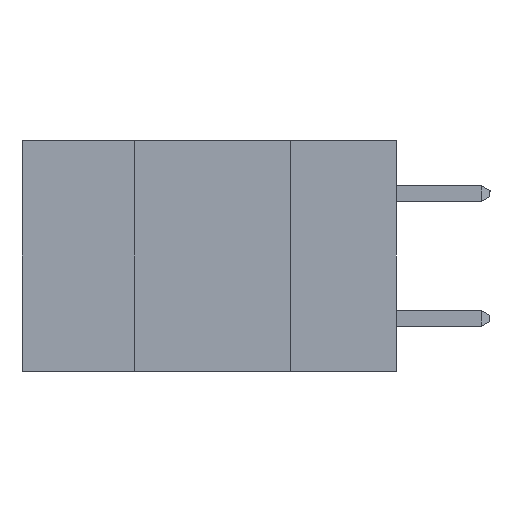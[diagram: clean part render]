
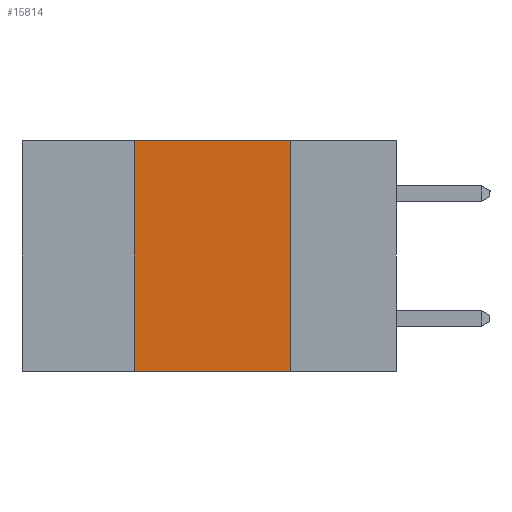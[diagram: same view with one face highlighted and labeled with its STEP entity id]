
A CAD part, left-side view. The second image highlights one B-rep face of the part: STEP entity #15814.
In plain terms, the highlighted planar face has unit normal (-1, 0, 0).
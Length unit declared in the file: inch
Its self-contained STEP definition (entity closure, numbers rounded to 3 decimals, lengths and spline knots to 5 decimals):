
#872 = EDGE_CURVE ( 'NONE', #3121, #7009, #13641, .T. ) ;
#1178 = LINE ( 'NONE', #25217, #14014 ) ;
#1834 = VECTOR ( 'NONE', #6778, 39.37008 ) ;
#2133 = ORIENTED_EDGE ( 'NONE', *, *, #15046, .F. ) ;
#2636 = CARTESIAN_POINT ( 'NONE',  ( 0., 0.6, 0. ) ) ;
#3121 = VERTEX_POINT ( 'NONE', #25473 ) ;
#3815 = LINE ( 'NONE', #19404, #4318 ) ;
#3816 = DIRECTION ( 'NONE',  ( 0., 0., 1. ) ) ;
#4318 = VECTOR ( 'NONE', #23713, 39.37008 ) ;
#5607 = EDGE_CURVE ( 'NONE', #24345, #25423, #3815, .T. ) ;
#6086 = CARTESIAN_POINT ( 'NONE',  ( 0., 0.42, 0. ) ) ;
#6778 = DIRECTION ( 'NONE',  ( 0., -1., 0. ) ) ;
#7009 = VERTEX_POINT ( 'NONE', #6086 ) ;
#7557 = ORIENTED_EDGE ( 'NONE', *, *, #872, .F. ) ;
#7639 = CARTESIAN_POINT ( 'NONE',  ( 0., 0.17, -0.37 ) ) ;
#7720 = ORIENTED_EDGE ( 'NONE', *, *, #5607, .F. ) ;
#7877 = PLANE ( 'NONE',  #23860 ) ;
#7921 = ORIENTED_EDGE ( 'NONE', *, *, #22756, .T. ) ;
#11538 = DIRECTION ( 'NONE',  ( 0., -1., 0. ) ) ;
#12291 = EDGE_LOOP ( 'NONE', ( #7720, #2133, #7557, #7921 ) ) ;
#13382 = CARTESIAN_POINT ( 'NONE',  ( 0., 0.42, -0.37 ) ) ;
#13641 = LINE ( 'NONE', #13382, #19537 ) ;
#14014 = VECTOR ( 'NONE', #11538, 39.37008 ) ;
#15046 = EDGE_CURVE ( 'NONE', #7009, #24345, #20687, .T. ) ;
#15814 = ADVANCED_FACE ( 'NONE', ( #21802 ), #7877, .F. ) ;
#18896 = CARTESIAN_POINT ( 'NONE',  ( 0., 0.17, 0. ) ) ;
#19404 = CARTESIAN_POINT ( 'NONE',  ( 0., 0.17, -0.37 ) ) ;
#19537 = VECTOR ( 'NONE', #3816, 39.37008 ) ;
#20687 = LINE ( 'NONE', #2636, #1834 ) ;
#21672 = CARTESIAN_POINT ( 'NONE',  ( 0., 0.6, 0. ) ) ;
#21802 = FACE_OUTER_BOUND ( 'NONE', #12291, .T. ) ;
#22059 = DIRECTION ( 'NONE',  ( 1., 0., 0. ) ) ;
#22756 = EDGE_CURVE ( 'NONE', #3121, #25423, #1178, .T. ) ;
#23635 = DIRECTION ( 'NONE',  ( 0., 0., -1. ) ) ;
#23713 = DIRECTION ( 'NONE',  ( 0., 0., -1. ) ) ;
#23860 = AXIS2_PLACEMENT_3D ( 'NONE', #21672, #22059, #23635 ) ;
#24345 = VERTEX_POINT ( 'NONE', #18896 ) ;
#25217 = CARTESIAN_POINT ( 'NONE',  ( 0., 0.6, -0.37 ) ) ;
#25423 = VERTEX_POINT ( 'NONE', #7639 ) ;
#25473 = CARTESIAN_POINT ( 'NONE',  ( 0., 0.42, -0.37 ) ) ;
